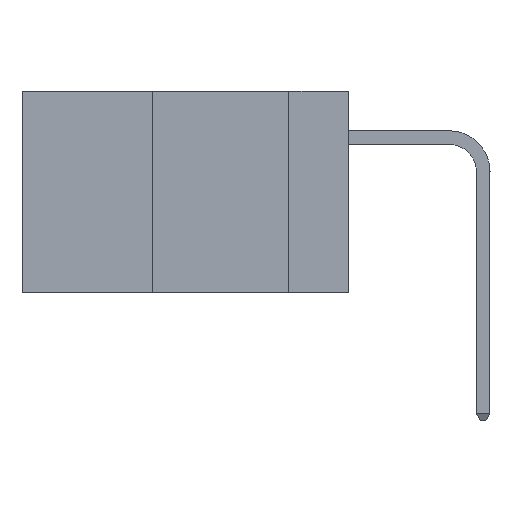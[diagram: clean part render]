
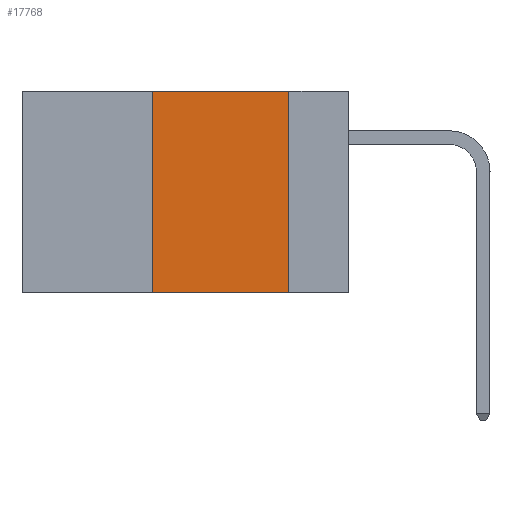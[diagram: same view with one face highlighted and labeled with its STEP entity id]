
A CAD part, left-side view. The second image highlights one B-rep face of the part: STEP entity #17768.
In plain terms, the highlighted planar face has unit normal (-1, 0, 0).
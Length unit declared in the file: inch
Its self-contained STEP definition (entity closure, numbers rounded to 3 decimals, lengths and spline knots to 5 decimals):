
#1430 = CARTESIAN_POINT ( 'NONE',  ( 0., 0.36, -0.37 ) ) ;
#1765 = ORIENTED_EDGE ( 'NONE', *, *, #6518, .F. ) ;
#2722 = VECTOR ( 'NONE', #32506, 39.37008 ) ;
#3705 = VECTOR ( 'NONE', #19349, 39.37008 ) ;
#6518 = EDGE_CURVE ( 'NONE', #36651, #13383, #20416, .T. ) ;
#7220 = EDGE_CURVE ( 'NONE', #15953, #35801, #9000, .T. ) ;
#7573 = CARTESIAN_POINT ( 'NONE',  ( 0., 0.36, 0. ) ) ;
#8065 = CARTESIAN_POINT ( 'NONE',  ( 0., 0.36, 0. ) ) ;
#8496 = PLANE ( 'NONE',  #11252 ) ;
#9000 = LINE ( 'NONE', #31690, #31089 ) ;
#10911 = EDGE_CURVE ( 'NONE', #13383, #15953, #19061, .T. ) ;
#11252 = AXIS2_PLACEMENT_3D ( 'NONE', #31547, #14307, #34432 ) ;
#12806 = VECTOR ( 'NONE', #16734, 39.37008 ) ;
#13383 = VERTEX_POINT ( 'NONE', #7573 ) ;
#14307 = DIRECTION ( 'NONE',  ( 1., 0., 0. ) ) ;
#15953 = VERTEX_POINT ( 'NONE', #21278 ) ;
#16734 = DIRECTION ( 'NONE',  ( 0., 0., 1. ) ) ;
#17768 = ADVANCED_FACE ( 'NONE', ( #24763 ), #8496, .F. ) ;
#19061 = LINE ( 'NONE', #33818, #3705 ) ;
#19349 = DIRECTION ( 'NONE',  ( 0., -1., 0. ) ) ;
#20416 = LINE ( 'NONE', #8065, #12806 ) ;
#21278 = CARTESIAN_POINT ( 'NONE',  ( 0., 0.11, 0. ) ) ;
#22240 = ORIENTED_EDGE ( 'NONE', *, *, #7220, .F. ) ;
#24763 = FACE_OUTER_BOUND ( 'NONE', #32919, .T. ) ;
#26727 = ORIENTED_EDGE ( 'NONE', *, *, #28251, .T. ) ;
#26845 = CARTESIAN_POINT ( 'NONE',  ( 0., 0.6, -0.37 ) ) ;
#28251 = EDGE_CURVE ( 'NONE', #36651, #35801, #32490, .T. ) ;
#28349 = CARTESIAN_POINT ( 'NONE',  ( 0., 0.11, -0.37 ) ) ;
#31089 = VECTOR ( 'NONE', #34571, 39.37008 ) ;
#31547 = CARTESIAN_POINT ( 'NONE',  ( 0., 0.6, 0. ) ) ;
#31690 = CARTESIAN_POINT ( 'NONE',  ( 0., 0.11, 0. ) ) ;
#32490 = LINE ( 'NONE', #26845, #2722 ) ;
#32506 = DIRECTION ( 'NONE',  ( 0., -1., 0. ) ) ;
#32919 = EDGE_LOOP ( 'NONE', ( #22240, #37395, #1765, #26727 ) ) ;
#33818 = CARTESIAN_POINT ( 'NONE',  ( 0., 0.6, 0. ) ) ;
#34432 = DIRECTION ( 'NONE',  ( 0., 0., -1. ) ) ;
#34571 = DIRECTION ( 'NONE',  ( 0., 0., -1. ) ) ;
#35801 = VERTEX_POINT ( 'NONE', #28349 ) ;
#36651 = VERTEX_POINT ( 'NONE', #1430 ) ;
#37395 = ORIENTED_EDGE ( 'NONE', *, *, #10911, .F. ) ;
